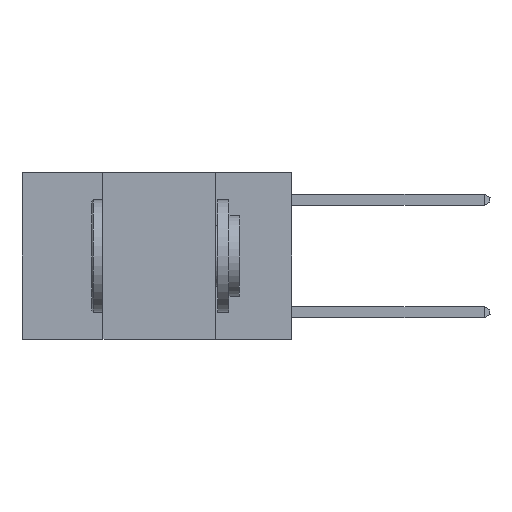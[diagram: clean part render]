
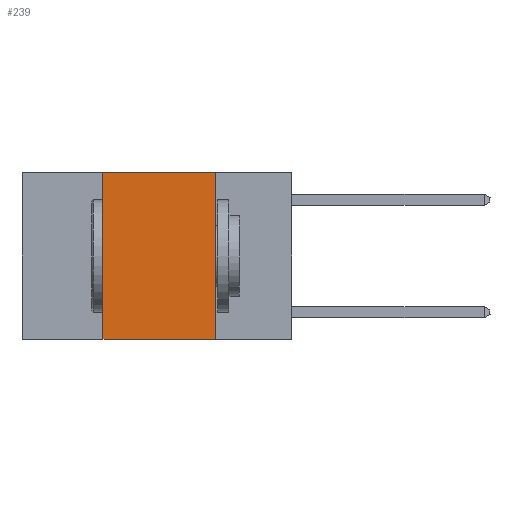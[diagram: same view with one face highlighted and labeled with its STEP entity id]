
A CAD part, left-side view. The second image highlights one B-rep face of the part: STEP entity #239.
In plain terms, the highlighted planar face has unit normal (-1, 0, 0).
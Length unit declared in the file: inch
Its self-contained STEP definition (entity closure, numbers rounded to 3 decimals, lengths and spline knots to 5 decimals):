
#239 = ADVANCED_FACE ( 'NONE', ( #1637 ), #12406, .F. ) ;
#604 = ORIENTED_EDGE ( 'NONE', *, *, #17727, .F. ) ;
#1334 = CARTESIAN_POINT ( 'NONE',  ( 0., 0.17, -0.37 ) ) ;
#1371 = ORIENTED_EDGE ( 'NONE', *, *, #6023, .F. ) ;
#1637 = FACE_OUTER_BOUND ( 'NONE', #9151, .T. ) ;
#2376 = EDGE_CURVE ( 'NONE', #11051, #17953, #7134, .T. ) ;
#2775 = DIRECTION ( 'NONE',  ( 0., -1., 0. ) ) ;
#3173 = VERTEX_POINT ( 'NONE', #14151 ) ;
#3337 = DIRECTION ( 'NONE',  ( 0., 0., -1. ) ) ;
#3352 = ORIENTED_EDGE ( 'NONE', *, *, #8625, .F. ) ;
#3857 = LINE ( 'NONE', #4048, #8826 ) ;
#4048 = CARTESIAN_POINT ( 'NONE',  ( 0., 0.42, 0. ) ) ;
#4703 = VECTOR ( 'NONE', #10551, 39.37008 ) ;
#4840 = CARTESIAN_POINT ( 'NONE',  ( 0., 0.6, 0. ) ) ;
#5800 = CARTESIAN_POINT ( 'NONE',  ( 0., 0.6, 0. ) ) ;
#6023 = EDGE_CURVE ( 'NONE', #18232, #17953, #6386, .T. ) ;
#6386 = LINE ( 'NONE', #7697, #12507 ) ;
#7134 = LINE ( 'NONE', #7324, #4703 ) ;
#7324 = CARTESIAN_POINT ( 'NONE',  ( 0., 0.6, -0.37 ) ) ;
#7697 = CARTESIAN_POINT ( 'NONE',  ( 0., 0.17, 0. ) ) ;
#7763 = DIRECTION ( 'NONE',  ( 1., 0., 0. ) ) ;
#8625 = EDGE_CURVE ( 'NONE', #3173, #18232, #10226, .T. ) ;
#8826 = VECTOR ( 'NONE', #19060, 39.37008 ) ;
#9151 = EDGE_LOOP ( 'NONE', ( #1371, #3352, #604, #12713 ) ) ;
#10226 = LINE ( 'NONE', #5800, #16398 ) ;
#10551 = DIRECTION ( 'NONE',  ( 0., -1., 0. ) ) ;
#11051 = VERTEX_POINT ( 'NONE', #11674 ) ;
#11674 = CARTESIAN_POINT ( 'NONE',  ( 0., 0.42, -0.37 ) ) ;
#12406 = PLANE ( 'NONE',  #12520 ) ;
#12507 = VECTOR ( 'NONE', #13846, 39.37008 ) ;
#12520 = AXIS2_PLACEMENT_3D ( 'NONE', #4840, #7763, #3337 ) ;
#12713 = ORIENTED_EDGE ( 'NONE', *, *, #2376, .T. ) ;
#13846 = DIRECTION ( 'NONE',  ( 0., 0., -1. ) ) ;
#14151 = CARTESIAN_POINT ( 'NONE',  ( 0., 0.42, 0. ) ) ;
#16398 = VECTOR ( 'NONE', #2775, 39.37008 ) ;
#17727 = EDGE_CURVE ( 'NONE', #11051, #3173, #3857, .T. ) ;
#17953 = VERTEX_POINT ( 'NONE', #1334 ) ;
#18232 = VERTEX_POINT ( 'NONE', #19626 ) ;
#19060 = DIRECTION ( 'NONE',  ( 0., 0., 1. ) ) ;
#19626 = CARTESIAN_POINT ( 'NONE',  ( 0., 0.17, 0. ) ) ;
